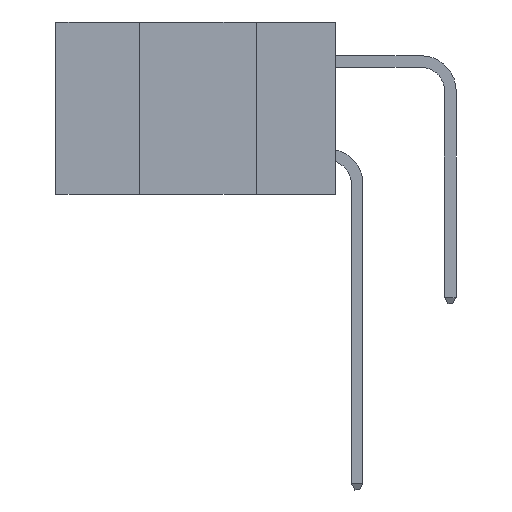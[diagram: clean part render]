
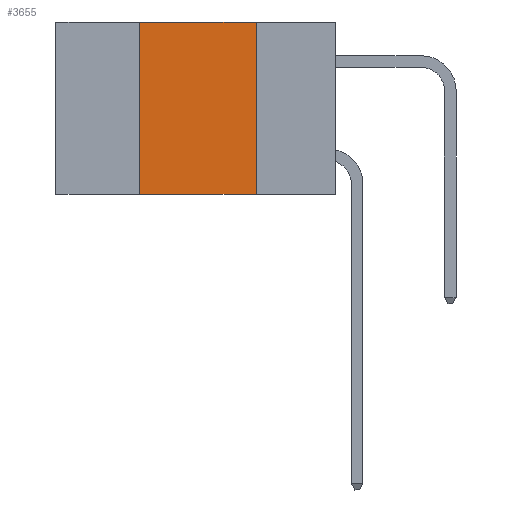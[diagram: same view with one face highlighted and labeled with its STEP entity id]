
A CAD part, left-side view. The second image highlights one B-rep face of the part: STEP entity #3655.
In plain terms, the highlighted planar face has unit normal (-1, 0, 0).
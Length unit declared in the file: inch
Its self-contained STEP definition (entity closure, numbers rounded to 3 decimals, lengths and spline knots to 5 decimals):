
#5 = EDGE_CURVE ( 'NONE', #8657, #6135, #2342, .T. ) ;
#33 = EDGE_CURVE ( 'NONE', #11481, #5095, #13050, .T. ) ;
#86 = EDGE_CURVE ( 'NONE', #11481, #6135, #6535, .T. ) ;
#1517 = DIRECTION ( 'NONE',  ( 1., 0., 0. ) ) ;
#2342 = LINE ( 'NONE', #5881, #13350 ) ;
#2533 = ORIENTED_EDGE ( 'NONE', *, *, #33, .F. ) ;
#3583 = CARTESIAN_POINT ( 'NONE',  ( 0., 0.17, 0. ) ) ;
#3617 = CARTESIAN_POINT ( 'NONE',  ( 0., 0.6, -0.37 ) ) ;
#3655 = ADVANCED_FACE ( 'NONE', ( #6199 ), #13185, .F. ) ;
#3834 = LINE ( 'NONE', #5504, #9353 ) ;
#4054 = EDGE_LOOP ( 'NONE', ( #7764, #13501, #2533, #8951 ) ) ;
#4654 = VECTOR ( 'NONE', #8854, 39.37008 ) ;
#5095 = VERTEX_POINT ( 'NONE', #6753 ) ;
#5504 = CARTESIAN_POINT ( 'NONE',  ( 0., 0.6, 0. ) ) ;
#5881 = CARTESIAN_POINT ( 'NONE',  ( 0., 0.17, 0. ) ) ;
#5930 = DIRECTION ( 'NONE',  ( 0., 0., -1. ) ) ;
#6135 = VERTEX_POINT ( 'NONE', #10587 ) ;
#6199 = FACE_OUTER_BOUND ( 'NONE', #4054, .T. ) ;
#6203 = VECTOR ( 'NONE', #9360, 39.37008 ) ;
#6535 = LINE ( 'NONE', #3617, #6203 ) ;
#6590 = DIRECTION ( 'NONE',  ( 0., -1., 0. ) ) ;
#6753 = CARTESIAN_POINT ( 'NONE',  ( 0., 0.42, 0. ) ) ;
#6940 = AXIS2_PLACEMENT_3D ( 'NONE', #7043, #1517, #9240 ) ;
#7043 = CARTESIAN_POINT ( 'NONE',  ( 0., 0.6, 0. ) ) ;
#7275 = CARTESIAN_POINT ( 'NONE',  ( 0., 0.42, -0.37 ) ) ;
#7720 = EDGE_CURVE ( 'NONE', #5095, #8657, #3834, .T. ) ;
#7764 = ORIENTED_EDGE ( 'NONE', *, *, #5, .F. ) ;
#8657 = VERTEX_POINT ( 'NONE', #3583 ) ;
#8854 = DIRECTION ( 'NONE',  ( 0., 0., 1. ) ) ;
#8951 = ORIENTED_EDGE ( 'NONE', *, *, #86, .T. ) ;
#9002 = CARTESIAN_POINT ( 'NONE',  ( 0., 0.42, 0. ) ) ;
#9240 = DIRECTION ( 'NONE',  ( 0., 0., -1. ) ) ;
#9353 = VECTOR ( 'NONE', #6590, 39.37008 ) ;
#9360 = DIRECTION ( 'NONE',  ( 0., -1., 0. ) ) ;
#10587 = CARTESIAN_POINT ( 'NONE',  ( 0., 0.17, -0.37 ) ) ;
#11481 = VERTEX_POINT ( 'NONE', #7275 ) ;
#13050 = LINE ( 'NONE', #9002, #4654 ) ;
#13185 = PLANE ( 'NONE',  #6940 ) ;
#13350 = VECTOR ( 'NONE', #5930, 39.37008 ) ;
#13501 = ORIENTED_EDGE ( 'NONE', *, *, #7720, .F. ) ;
